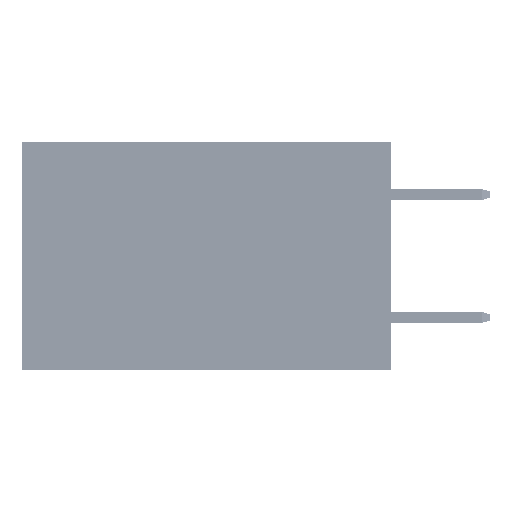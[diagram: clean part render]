
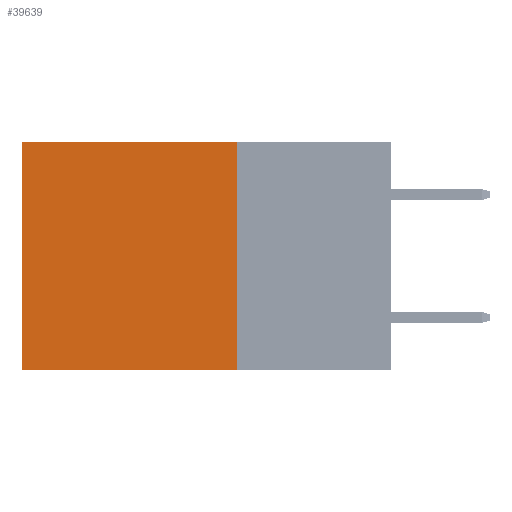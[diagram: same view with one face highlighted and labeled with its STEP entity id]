
A CAD part, left-side view. The second image highlights one B-rep face of the part: STEP entity #39639.
In plain terms, the highlighted planar face has unit normal (-1, 0, 0).
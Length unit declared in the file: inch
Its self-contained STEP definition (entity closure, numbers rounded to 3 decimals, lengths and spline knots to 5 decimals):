
#141 = DIRECTION ( 'NONE',  ( 0., 0., -1. ) ) ;
#326 = CARTESIAN_POINT ( 'NONE',  ( 0.2875, 0.6, -0.37 ) ) ;
#2075 = VERTEX_POINT ( 'NONE', #41899 ) ;
#4834 = DIRECTION ( 'NONE',  ( 1., 0., 0. ) ) ;
#4988 = EDGE_CURVE ( 'NONE', #38271, #27747, #36978, .T. ) ;
#6575 = ORIENTED_EDGE ( 'NONE', *, *, #12799, .T. ) ;
#7477 = CARTESIAN_POINT ( 'NONE',  ( 0.2875, 0.6, 0. ) ) ;
#7988 = DIRECTION ( 'NONE',  ( 0., 1., 0. ) ) ;
#8181 = LINE ( 'NONE', #9950, #17777 ) ;
#8320 = EDGE_CURVE ( 'NONE', #27350, #2075, #8181, .T. ) ;
#9950 = CARTESIAN_POINT ( 'NONE',  ( 0.2875, 0.25, 0. ) ) ;
#10864 = VECTOR ( 'NONE', #25727, 39.37008 ) ;
#11502 = DIRECTION ( 'NONE',  ( 0., 0., -1. ) ) ;
#11959 = CARTESIAN_POINT ( 'NONE',  ( 0.2875, 0.25, 0. ) ) ;
#12799 = EDGE_CURVE ( 'NONE', #27350, #38271, #24534, .T. ) ;
#14739 = DIRECTION ( 'NONE',  ( 0., 0., -1. ) ) ;
#14795 = EDGE_LOOP ( 'NONE', ( #19053, #20503, #29564, #6575 ) ) ;
#14876 = AXIS2_PLACEMENT_3D ( 'NONE', #11959, #4834, #11502 ) ;
#17777 = VECTOR ( 'NONE', #141, 39.37008 ) ;
#19053 = ORIENTED_EDGE ( 'NONE', *, *, #4988, .T. ) ;
#20503 = ORIENTED_EDGE ( 'NONE', *, *, #42144, .F. ) ;
#21158 = VECTOR ( 'NONE', #7988, 39.37008 ) ;
#21977 = CARTESIAN_POINT ( 'NONE',  ( 0.2875, 0.25, -0.37 ) ) ;
#24534 = LINE ( 'NONE', #40106, #21158 ) ;
#25112 = VECTOR ( 'NONE', #14739, 39.37008 ) ;
#25727 = DIRECTION ( 'NONE',  ( 0., 1., 0. ) ) ;
#26085 = PLANE ( 'NONE',  #14876 ) ;
#27350 = VERTEX_POINT ( 'NONE', #42110 ) ;
#27747 = VERTEX_POINT ( 'NONE', #326 ) ;
#29564 = ORIENTED_EDGE ( 'NONE', *, *, #8320, .F. ) ;
#32017 = CARTESIAN_POINT ( 'NONE',  ( 0.2875, 0.6, 0. ) ) ;
#35101 = LINE ( 'NONE', #21977, #10864 ) ;
#36978 = LINE ( 'NONE', #7477, #25112 ) ;
#38271 = VERTEX_POINT ( 'NONE', #32017 ) ;
#39210 = FACE_OUTER_BOUND ( 'NONE', #14795, .T. ) ;
#39639 = ADVANCED_FACE ( 'NONE', ( #39210 ), #26085, .F. ) ;
#40106 = CARTESIAN_POINT ( 'NONE',  ( 0.2875, 0.25, 0. ) ) ;
#41899 = CARTESIAN_POINT ( 'NONE',  ( 0.2875, 0.25, -0.37 ) ) ;
#42110 = CARTESIAN_POINT ( 'NONE',  ( 0.2875, 0.25, 0. ) ) ;
#42144 = EDGE_CURVE ( 'NONE', #2075, #27747, #35101, .T. ) ;
